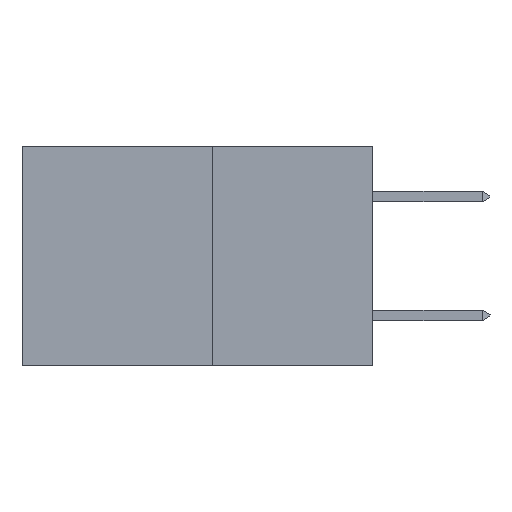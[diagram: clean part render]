
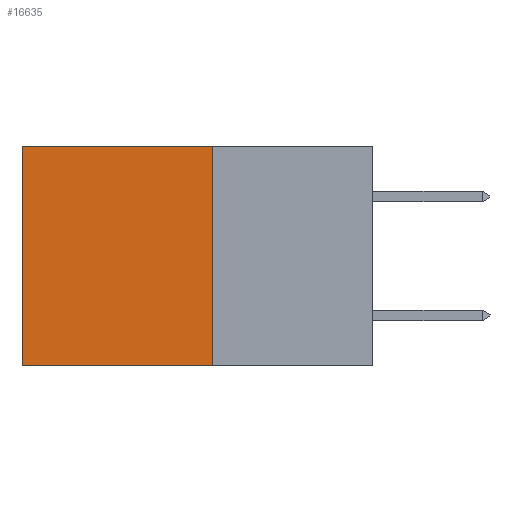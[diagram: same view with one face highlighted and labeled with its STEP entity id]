
A CAD part, left-side view. The second image highlights one B-rep face of the part: STEP entity #16635.
In plain terms, the highlighted planar face has unit normal (-1, 0, 0).
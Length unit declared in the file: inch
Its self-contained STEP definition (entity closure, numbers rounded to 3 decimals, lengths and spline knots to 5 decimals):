
#86 = CARTESIAN_POINT ( 'NONE',  ( 0.277, 0.27, -0.37 ) ) ;
#296 = CARTESIAN_POINT ( 'NONE',  ( 0.277, 0.59, 0. ) ) ;
#2719 = ORIENTED_EDGE ( 'NONE', *, *, #7440, .T. ) ;
#3310 = VERTEX_POINT ( 'NONE', #18304 ) ;
#5154 = CARTESIAN_POINT ( 'NONE',  ( 0.277, 0.59, -0.37 ) ) ;
#6857 = PLANE ( 'NONE',  #23110 ) ;
#6948 = ORIENTED_EDGE ( 'NONE', *, *, #15479, .F. ) ;
#7440 = EDGE_CURVE ( 'NONE', #3310, #12108, #11965, .T. ) ;
#8186 = VERTEX_POINT ( 'NONE', #10372 ) ;
#8969 = LINE ( 'NONE', #23113, #18601 ) ;
#9924 = VECTOR ( 'NONE', #21452, 39.37008 ) ;
#10108 = DIRECTION ( 'NONE',  ( 0., 0., -1. ) ) ;
#10183 = CARTESIAN_POINT ( 'NONE',  ( 0.277, 0.27, -0.37 ) ) ;
#10372 = CARTESIAN_POINT ( 'NONE',  ( 0.277, 0.59, -0.37 ) ) ;
#10511 = DIRECTION ( 'NONE',  ( 1., 0., 0. ) ) ;
#10923 = EDGE_LOOP ( 'NONE', ( #22621, #22928, #6948, #2719 ) ) ;
#11965 = LINE ( 'NONE', #14849, #21008 ) ;
#12108 = VERTEX_POINT ( 'NONE', #296 ) ;
#14849 = CARTESIAN_POINT ( 'NONE',  ( 0.277, 0.27, 0. ) ) ;
#15479 = EDGE_CURVE ( 'NONE', #3310, #20031, #19428, .T. ) ;
#15699 = FACE_OUTER_BOUND ( 'NONE', #10923, .T. ) ;
#15955 = EDGE_CURVE ( 'NONE', #20031, #8186, #8969, .T. ) ;
#16635 = ADVANCED_FACE ( 'NONE', ( #15699 ), #6857, .F. ) ;
#17732 = DIRECTION ( 'NONE',  ( 0., 1., 0. ) ) ;
#18304 = CARTESIAN_POINT ( 'NONE',  ( 0.277, 0.27, 0. ) ) ;
#18601 = VECTOR ( 'NONE', #21274, 39.37008 ) ;
#19174 = EDGE_CURVE ( 'NONE', #12108, #8186, #20102, .T. ) ;
#19428 = LINE ( 'NONE', #10183, #23022 ) ;
#20031 = VERTEX_POINT ( 'NONE', #86 ) ;
#20102 = LINE ( 'NONE', #5154, #9924 ) ;
#21008 = VECTOR ( 'NONE', #17732, 39.37008 ) ;
#21274 = DIRECTION ( 'NONE',  ( 0., 1., 0. ) ) ;
#21317 = CARTESIAN_POINT ( 'NONE',  ( 0.277, 0.27, -0.37 ) ) ;
#21452 = DIRECTION ( 'NONE',  ( 0., 0., -1. ) ) ;
#22621 = ORIENTED_EDGE ( 'NONE', *, *, #19174, .T. ) ;
#22928 = ORIENTED_EDGE ( 'NONE', *, *, #15955, .F. ) ;
#23022 = VECTOR ( 'NONE', #10108, 39.37008 ) ;
#23082 = DIRECTION ( 'NONE',  ( 0., 0., -1. ) ) ;
#23110 = AXIS2_PLACEMENT_3D ( 'NONE', #21317, #10511, #23082 ) ;
#23113 = CARTESIAN_POINT ( 'NONE',  ( 0.277, 0.27, -0.37 ) ) ;
